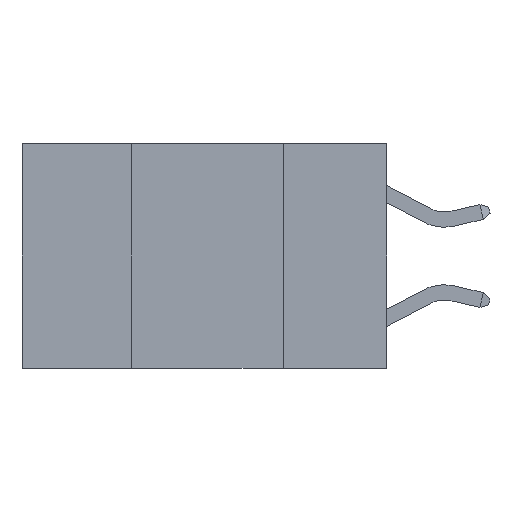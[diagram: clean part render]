
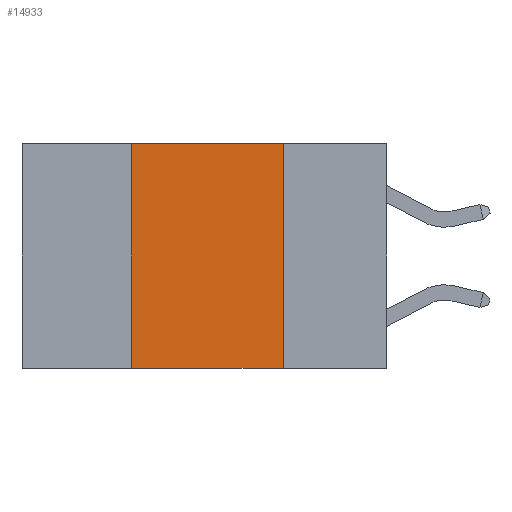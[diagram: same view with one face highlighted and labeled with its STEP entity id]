
A CAD part, left-side view. The second image highlights one B-rep face of the part: STEP entity #14933.
In plain terms, the highlighted planar face has unit normal (-1, 0, 0).
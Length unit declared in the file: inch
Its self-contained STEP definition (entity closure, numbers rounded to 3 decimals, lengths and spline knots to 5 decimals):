
#2893 = EDGE_CURVE ( 'NONE', #29380, #15320, #28148, .T. ) ;
#3409 = CARTESIAN_POINT ( 'NONE',  ( 0., 0.6, 0. ) ) ;
#3768 = DIRECTION ( 'NONE',  ( 0., 0., -1. ) ) ;
#4422 = VECTOR ( 'NONE', #24916, 39.37008 ) ;
#6073 = PLANE ( 'NONE',  #20036 ) ;
#6196 = LINE ( 'NONE', #6340, #4422 ) ;
#6340 = CARTESIAN_POINT ( 'NONE',  ( 0., 0.17, 0. ) ) ;
#7720 = DIRECTION ( 'NONE',  ( 0., -1., 0. ) ) ;
#9572 = VERTEX_POINT ( 'NONE', #16446 ) ;
#9607 = VECTOR ( 'NONE', #28425, 39.37008 ) ;
#9907 = LINE ( 'NONE', #19426, #16544 ) ;
#11894 = LINE ( 'NONE', #14365, #9607 ) ;
#12822 = DIRECTION ( 'NONE',  ( 1., 0., 0. ) ) ;
#14032 = ORIENTED_EDGE ( 'NONE', *, *, #26707, .T. ) ;
#14365 = CARTESIAN_POINT ( 'NONE',  ( 0., 0.42, 0. ) ) ;
#14933 = ADVANCED_FACE ( 'NONE', ( #27060 ), #6073, .F. ) ;
#15177 = VERTEX_POINT ( 'NONE', #26408 ) ;
#15320 = VERTEX_POINT ( 'NONE', #25020 ) ;
#16446 = CARTESIAN_POINT ( 'NONE',  ( 0., 0.17, -0.37 ) ) ;
#16544 = VECTOR ( 'NONE', #7720, 39.37008 ) ;
#16573 = CARTESIAN_POINT ( 'NONE',  ( 0., 0.42, 0. ) ) ;
#16876 = EDGE_CURVE ( 'NONE', #15320, #9572, #6196, .T. ) ;
#17631 = CARTESIAN_POINT ( 'NONE',  ( 0., 0.6, 0. ) ) ;
#19426 = CARTESIAN_POINT ( 'NONE',  ( 0., 0.6, -0.37 ) ) ;
#20036 = AXIS2_PLACEMENT_3D ( 'NONE', #17631, #12822, #3768 ) ;
#20659 = VECTOR ( 'NONE', #24318, 39.37008 ) ;
#22331 = ORIENTED_EDGE ( 'NONE', *, *, #16876, .F. ) ;
#22639 = ORIENTED_EDGE ( 'NONE', *, *, #24958, .F. ) ;
#24318 = DIRECTION ( 'NONE',  ( 0., -1., 0. ) ) ;
#24916 = DIRECTION ( 'NONE',  ( 0., 0., -1. ) ) ;
#24958 = EDGE_CURVE ( 'NONE', #15177, #29380, #11894, .T. ) ;
#25020 = CARTESIAN_POINT ( 'NONE',  ( 0., 0.17, 0. ) ) ;
#26407 = ORIENTED_EDGE ( 'NONE', *, *, #2893, .F. ) ;
#26408 = CARTESIAN_POINT ( 'NONE',  ( 0., 0.42, -0.37 ) ) ;
#26707 = EDGE_CURVE ( 'NONE', #15177, #9572, #9907, .T. ) ;
#27060 = FACE_OUTER_BOUND ( 'NONE', #29704, .T. ) ;
#28148 = LINE ( 'NONE', #3409, #20659 ) ;
#28425 = DIRECTION ( 'NONE',  ( 0., 0., 1. ) ) ;
#29380 = VERTEX_POINT ( 'NONE', #16573 ) ;
#29704 = EDGE_LOOP ( 'NONE', ( #22331, #26407, #22639, #14032 ) ) ;
